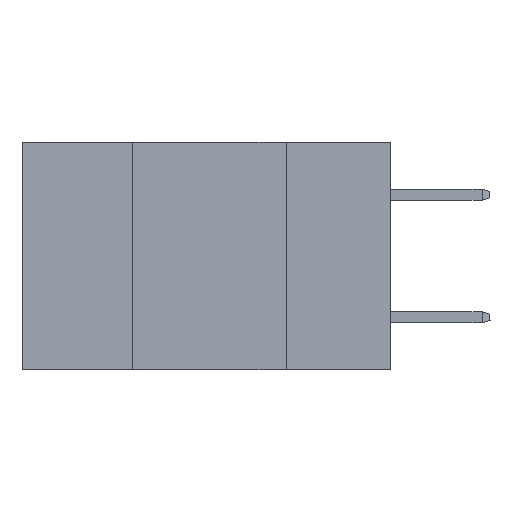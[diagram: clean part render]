
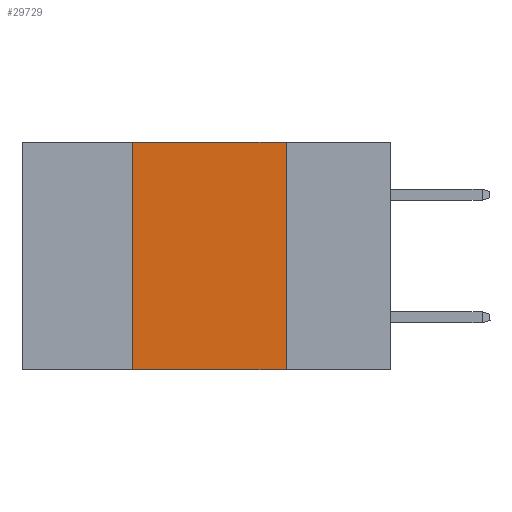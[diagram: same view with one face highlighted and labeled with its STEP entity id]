
A CAD part, left-side view. The second image highlights one B-rep face of the part: STEP entity #29729.
In plain terms, the highlighted planar face has unit normal (-1, 0, 0).
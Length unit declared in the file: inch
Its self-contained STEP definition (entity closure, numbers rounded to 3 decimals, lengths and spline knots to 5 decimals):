
#1291 = ORIENTED_EDGE ( 'NONE', *, *, #21463, .F. ) ;
#2175 = CARTESIAN_POINT ( 'NONE',  ( 0., 0.17, 0. ) ) ;
#7236 = VECTOR ( 'NONE', #20788, 39.37008 ) ;
#9308 = CARTESIAN_POINT ( 'NONE',  ( 0., 0.42, 0. ) ) ;
#12909 = CARTESIAN_POINT ( 'NONE',  ( 0., 0.17, 0. ) ) ;
#13447 = EDGE_CURVE ( 'NONE', #32488, #31087, #32895, .T. ) ;
#14656 = VECTOR ( 'NONE', #32784, 39.37008 ) ;
#15063 = VERTEX_POINT ( 'NONE', #25823 ) ;
#15509 = EDGE_CURVE ( 'NONE', #39647, #31087, #29289, .T. ) ;
#16565 = DIRECTION ( 'NONE',  ( 0., 0., -1. ) ) ;
#17261 = CARTESIAN_POINT ( 'NONE',  ( 0., 0.6, 0. ) ) ;
#17863 = DIRECTION ( 'NONE',  ( 0., -1., 0. ) ) ;
#18112 = DIRECTION ( 'NONE',  ( 0., 0., -1. ) ) ;
#20788 = DIRECTION ( 'NONE',  ( 0., -1., 0. ) ) ;
#21463 = EDGE_CURVE ( 'NONE', #15063, #32488, #25097, .T. ) ;
#22266 = CARTESIAN_POINT ( 'NONE',  ( 0., 0.42, -0.37 ) ) ;
#24560 = ORIENTED_EDGE ( 'NONE', *, *, #33453, .F. ) ;
#25097 = LINE ( 'NONE', #17261, #7236 ) ;
#25823 = CARTESIAN_POINT ( 'NONE',  ( 0., 0.42, 0. ) ) ;
#26820 = AXIS2_PLACEMENT_3D ( 'NONE', #31463, #38203, #18112 ) ;
#27159 = VECTOR ( 'NONE', #16565, 39.37008 ) ;
#29289 = LINE ( 'NONE', #40895, #37183 ) ;
#29293 = ORIENTED_EDGE ( 'NONE', *, *, #15509, .T. ) ;
#29696 = EDGE_LOOP ( 'NONE', ( #37655, #1291, #24560, #29293 ) ) ;
#29729 = ADVANCED_FACE ( 'NONE', ( #31228 ), #38765, .F. ) ;
#31087 = VERTEX_POINT ( 'NONE', #35006 ) ;
#31228 = FACE_OUTER_BOUND ( 'NONE', #29696, .T. ) ;
#31463 = CARTESIAN_POINT ( 'NONE',  ( 0., 0.6, 0. ) ) ;
#32488 = VERTEX_POINT ( 'NONE', #2175 ) ;
#32784 = DIRECTION ( 'NONE',  ( 0., 0., 1. ) ) ;
#32895 = LINE ( 'NONE', #12909, #27159 ) ;
#33453 = EDGE_CURVE ( 'NONE', #39647, #15063, #42939, .T. ) ;
#35006 = CARTESIAN_POINT ( 'NONE',  ( 0., 0.17, -0.37 ) ) ;
#37183 = VECTOR ( 'NONE', #17863, 39.37008 ) ;
#37655 = ORIENTED_EDGE ( 'NONE', *, *, #13447, .F. ) ;
#38203 = DIRECTION ( 'NONE',  ( 1., 0., 0. ) ) ;
#38765 = PLANE ( 'NONE',  #26820 ) ;
#39647 = VERTEX_POINT ( 'NONE', #22266 ) ;
#40895 = CARTESIAN_POINT ( 'NONE',  ( 0., 0.6, -0.37 ) ) ;
#42939 = LINE ( 'NONE', #9308, #14656 ) ;
